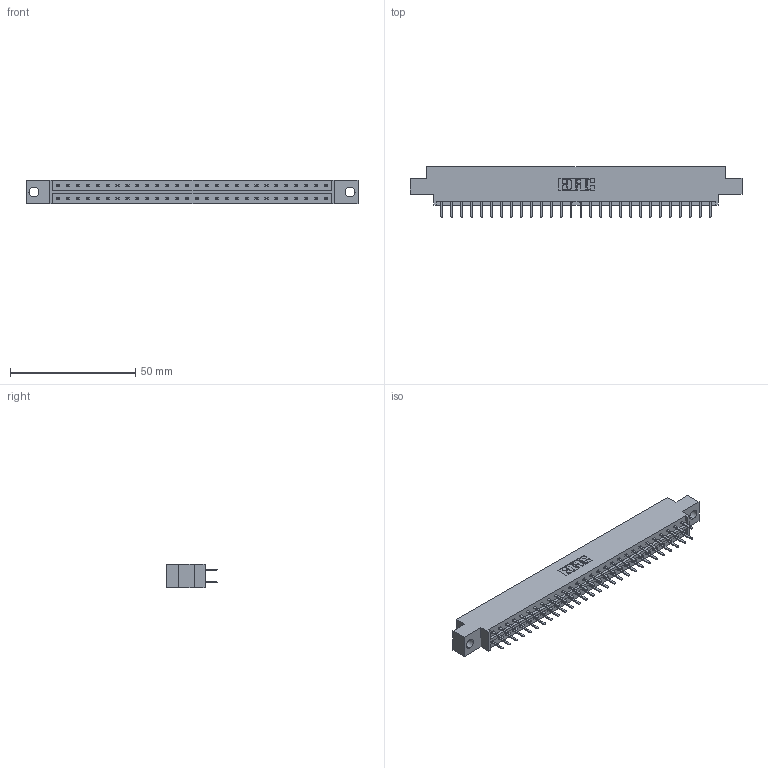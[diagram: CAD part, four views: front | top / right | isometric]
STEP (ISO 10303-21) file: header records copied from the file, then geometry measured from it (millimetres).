
FILE_DESCRIPTION (( 'STEP AP203' ), '1' );
FILE_NAME ('833-056-520-804.STEP', '2020-06-04T22:11:53', ( '' ), ( '' ), 'SwSTEP 2.0', 'SolidWorks 2020', '' );
FILE_SCHEMA (( 'CONFIG_CONTROL_DESIGN' ));
Length unit declared in the file: inch
Products named in the file (3): 833 Part_Offset - .156 Dia - TH; 833-056-520-804; 345-292-001_345-293-120
Assembly tree (57 placements, depth 2):
  833-056-520-804
    833 Part_Offset - .156 Dia - TH
    345-292-001_345-293-120  x56
Bounding box: 132.49 x 20.02 x 9.4 mm (x, y, z)
Volume: 13054.9 mm3; surface area: 15238.8 mm2
Topology: 57 solids, 57 shells, 3254 faces, 9451 edges, 6150 vertices
Faces by surface type: plane 2202, cylinder 1052
Entity records: 20073 total; most frequent: CARTESIAN_POINT 3358, ORIENTED_EDGE 3282, DIRECTION 2881, EDGE_CURVE 1641, VECTOR 1509, LINE 1509, VERTEX_POINT 1090, AXIS2_PLACEMENT_3D 686
